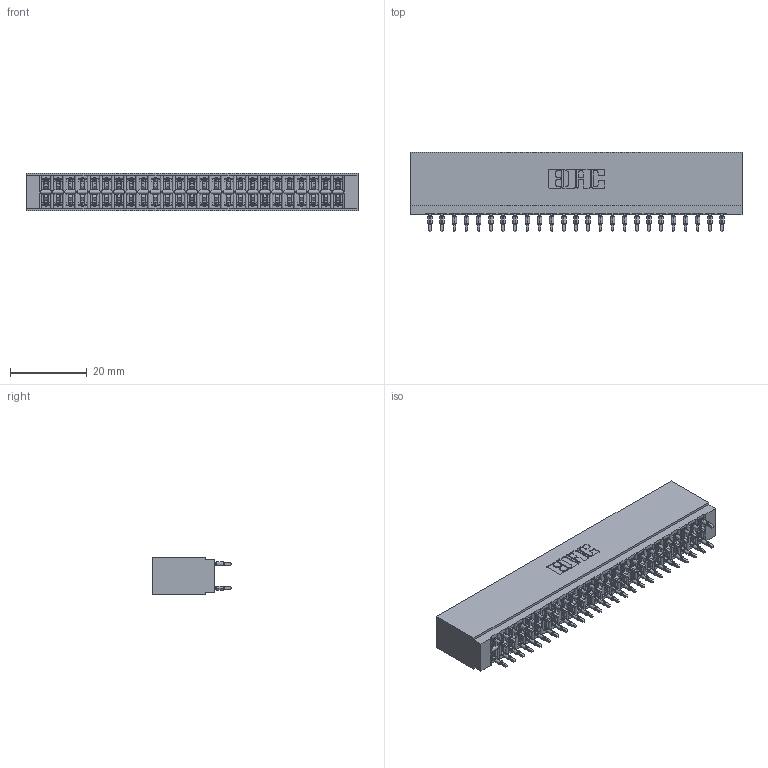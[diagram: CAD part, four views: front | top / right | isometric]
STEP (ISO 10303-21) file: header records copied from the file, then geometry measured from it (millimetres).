
FILE_DESCRIPTION (( 'STEP AP203' ), '1' );
FILE_NAME ('746-050-560-201.STEP', '2026-02-27T18:56:14', ( '' ), ( '' ), 'SwSTEP 2.0', 'SolidWorks 2023', '' );
FILE_SCHEMA (( 'CONFIG_CONTROL_DESIGN' ));
Length unit declared in the file: millimetre
Products named in the file (3): 746-292-001_560; 746 Part_.515 Slot Depth - 01; 746-050-560-201
Assembly tree (51 placements, depth 2):
  746-050-560-201
    746 Part_.515 Slot Depth - 01
    746-292-001_560  x50
Bounding box: 86.61 x 20.82 x 9.91 mm (x, y, z)
Volume: 9566.7 mm3; surface area: 15836.2 mm2
Topology: 51 solids, 51 shells, 4822 faces, 13413 edges, 8600 vertices
Faces by surface type: plane 2405, cylinder 1117, bspline 1000, torus 300
Entity records: 41166 total; most frequent: CARTESIAN_POINT 8329, ORIENTED_EDGE 7030, DIRECTION 5905, EDGE_CURVE 3515, LINE 3073, VECTOR 3073, VERTEX_POINT 2328, AXIS2_PLACEMENT_3D 1416
